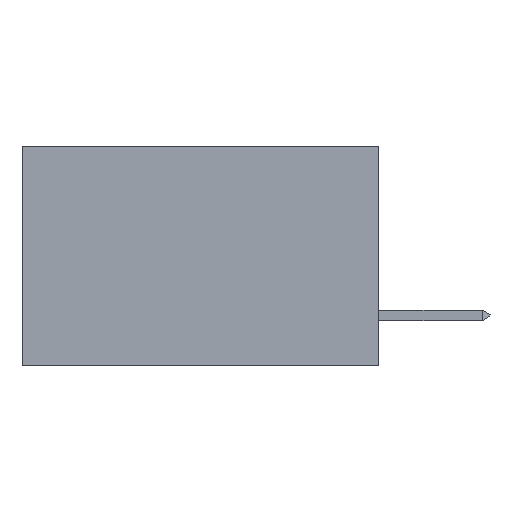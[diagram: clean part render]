
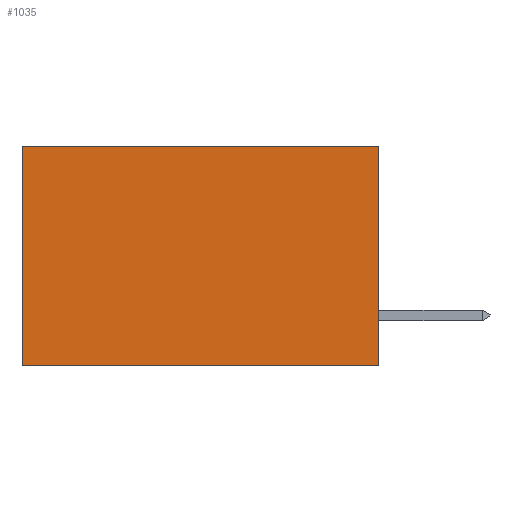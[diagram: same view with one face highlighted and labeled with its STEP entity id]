
A CAD part, left-side view. The second image highlights one B-rep face of the part: STEP entity #1035.
In plain terms, the highlighted planar face has unit normal (-1, 0, 0).
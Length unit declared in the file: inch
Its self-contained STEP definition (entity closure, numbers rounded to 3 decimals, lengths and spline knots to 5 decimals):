
#690 = CARTESIAN_POINT ( 'NONE',  ( 0.298, 0., 0. ) ) ;
#1035 = ADVANCED_FACE ( 'NONE', ( #12387 ), #12581, .F. ) ;
#1547 = CARTESIAN_POINT ( 'NONE',  ( 0.298, 0., 0. ) ) ;
#1683 = ORIENTED_EDGE ( 'NONE', *, *, #12119, .F. ) ;
#1809 = DIRECTION ( 'NONE',  ( 0., 1., 0. ) ) ;
#2056 = VECTOR ( 'NONE', #14229, 39.37008 ) ;
#2422 = VERTEX_POINT ( 'NONE', #10749 ) ;
#2542 = VERTEX_POINT ( 'NONE', #3435 ) ;
#2603 = VECTOR ( 'NONE', #14215, 39.37008 ) ;
#3435 = CARTESIAN_POINT ( 'NONE',  ( 0.298, 0., -0.37 ) ) ;
#3744 = DIRECTION ( 'NONE',  ( 1., 0., 0. ) ) ;
#4327 = CARTESIAN_POINT ( 'NONE',  ( 0.298, 0., -0.37 ) ) ;
#4768 = VECTOR ( 'NONE', #13733, 39.37008 ) ;
#4880 = CARTESIAN_POINT ( 'NONE',  ( 0.298, 0.6, 0. ) ) ;
#6005 = VECTOR ( 'NONE', #1809, 39.37008 ) ;
#6013 = ORIENTED_EDGE ( 'NONE', *, *, #13262, .F. ) ;
#6091 = LINE ( 'NONE', #4327, #2603 ) ;
#6426 = LINE ( 'NONE', #14375, #2056 ) ;
#7098 = ORIENTED_EDGE ( 'NONE', *, *, #8890, .T. ) ;
#7103 = DIRECTION ( 'NONE',  ( 0., 0., -1. ) ) ;
#8650 = EDGE_LOOP ( 'NONE', ( #13085, #1683, #6013, #7098 ) ) ;
#8830 = EDGE_CURVE ( 'NONE', #2422, #13307, #10742, .T. ) ;
#8890 = EDGE_CURVE ( 'NONE', #12039, #2422, #9155, .T. ) ;
#9155 = LINE ( 'NONE', #690, #6005 ) ;
#10458 = CARTESIAN_POINT ( 'NONE',  ( 0.298, 0., 0. ) ) ;
#10742 = LINE ( 'NONE', #4880, #4768 ) ;
#10749 = CARTESIAN_POINT ( 'NONE',  ( 0.298, 0.6, 0. ) ) ;
#12039 = VERTEX_POINT ( 'NONE', #1547 ) ;
#12119 = EDGE_CURVE ( 'NONE', #2542, #13307, #6091, .T. ) ;
#12387 = FACE_OUTER_BOUND ( 'NONE', #8650, .T. ) ;
#12581 = PLANE ( 'NONE',  #14476 ) ;
#13085 = ORIENTED_EDGE ( 'NONE', *, *, #8830, .T. ) ;
#13262 = EDGE_CURVE ( 'NONE', #12039, #2542, #6426, .T. ) ;
#13307 = VERTEX_POINT ( 'NONE', #14330 ) ;
#13733 = DIRECTION ( 'NONE',  ( 0., 0., -1. ) ) ;
#14215 = DIRECTION ( 'NONE',  ( 0., 1., 0. ) ) ;
#14229 = DIRECTION ( 'NONE',  ( 0., 0., -1. ) ) ;
#14330 = CARTESIAN_POINT ( 'NONE',  ( 0.298, 0.6, -0.37 ) ) ;
#14375 = CARTESIAN_POINT ( 'NONE',  ( 0.298, 0., 0. ) ) ;
#14476 = AXIS2_PLACEMENT_3D ( 'NONE', #10458, #3744, #7103 ) ;
